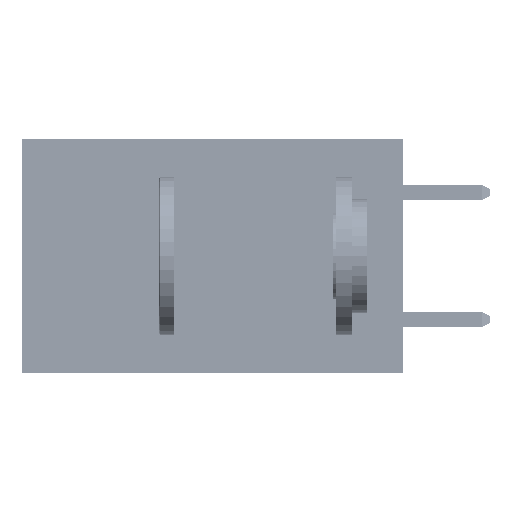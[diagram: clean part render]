
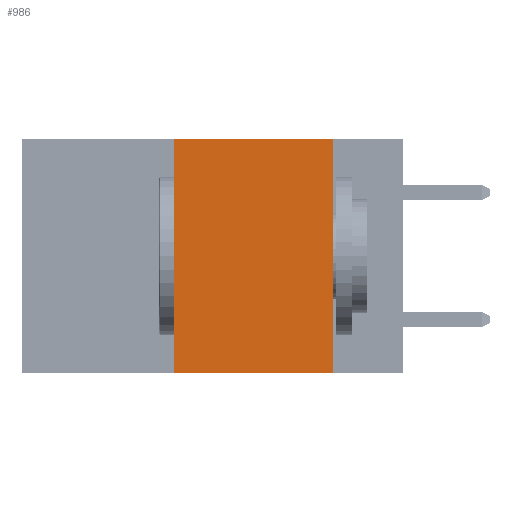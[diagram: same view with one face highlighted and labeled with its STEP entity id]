
A CAD part, left-side view. The second image highlights one B-rep face of the part: STEP entity #986.
In plain terms, the highlighted planar face has unit normal (-1, 0, 0).
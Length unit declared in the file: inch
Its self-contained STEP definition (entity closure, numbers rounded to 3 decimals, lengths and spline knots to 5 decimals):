
#96 = CARTESIAN_POINT ( 'NONE',  ( 0., 0.6, -0.37 ) ) ;
#986 = ADVANCED_FACE ( 'NONE', ( #22751 ), #46967, .F. ) ;
#1031 = DIRECTION ( 'NONE',  ( 1., 0., 0. ) ) ;
#2499 = EDGE_CURVE ( 'NONE', #31330, #11878, #14927, .T. ) ;
#3254 = CARTESIAN_POINT ( 'NONE',  ( 0., 0.36, -0.37 ) ) ;
#4270 = VECTOR ( 'NONE', #18040, 39.37008 ) ;
#5153 = VECTOR ( 'NONE', #24716, 39.37008 ) ;
#6411 = ORIENTED_EDGE ( 'NONE', *, *, #33338, .F. ) ;
#6518 = EDGE_CURVE ( 'NONE', #32225, #39727, #40614, .T. ) ;
#9819 = DIRECTION ( 'NONE',  ( 0., 0., -1. ) ) ;
#11649 = AXIS2_PLACEMENT_3D ( 'NONE', #13761, #1031, #9819 ) ;
#11878 = VERTEX_POINT ( 'NONE', #40373 ) ;
#13761 = CARTESIAN_POINT ( 'NONE',  ( 0., 0.6, 0. ) ) ;
#14102 = EDGE_CURVE ( 'NONE', #39727, #11878, #18438, .T. ) ;
#14927 = LINE ( 'NONE', #96, #43961 ) ;
#15981 = ORIENTED_EDGE ( 'NONE', *, *, #2499, .T. ) ;
#18040 = DIRECTION ( 'NONE',  ( 0., 0., -1. ) ) ;
#18438 = LINE ( 'NONE', #26882, #4270 ) ;
#19291 = VECTOR ( 'NONE', #24518, 39.37008 ) ;
#22751 = FACE_OUTER_BOUND ( 'NONE', #25997, .T. ) ;
#24518 = DIRECTION ( 'NONE',  ( 0., 0., 1. ) ) ;
#24716 = DIRECTION ( 'NONE',  ( 0., -1., 0. ) ) ;
#25997 = EDGE_LOOP ( 'NONE', ( #36776, #30763, #6411, #15981 ) ) ;
#26882 = CARTESIAN_POINT ( 'NONE',  ( 0., 0.11, 0. ) ) ;
#28959 = LINE ( 'NONE', #37113, #19291 ) ;
#29758 = CARTESIAN_POINT ( 'NONE',  ( 0., 0.36, 0. ) ) ;
#30763 = ORIENTED_EDGE ( 'NONE', *, *, #6518, .F. ) ;
#31330 = VERTEX_POINT ( 'NONE', #3254 ) ;
#32225 = VERTEX_POINT ( 'NONE', #29758 ) ;
#33338 = EDGE_CURVE ( 'NONE', #31330, #32225, #28959, .T. ) ;
#36776 = ORIENTED_EDGE ( 'NONE', *, *, #14102, .F. ) ;
#37113 = CARTESIAN_POINT ( 'NONE',  ( 0., 0.36, 0. ) ) ;
#37133 = CARTESIAN_POINT ( 'NONE',  ( 0., 0.6, 0. ) ) ;
#39727 = VERTEX_POINT ( 'NONE', #48121 ) ;
#40373 = CARTESIAN_POINT ( 'NONE',  ( 0., 0.11, -0.37 ) ) ;
#40614 = LINE ( 'NONE', #37133, #5153 ) ;
#43961 = VECTOR ( 'NONE', #44952, 39.37008 ) ;
#44952 = DIRECTION ( 'NONE',  ( 0., -1., 0. ) ) ;
#46967 = PLANE ( 'NONE',  #11649 ) ;
#48121 = CARTESIAN_POINT ( 'NONE',  ( 0., 0.11, 0. ) ) ;
